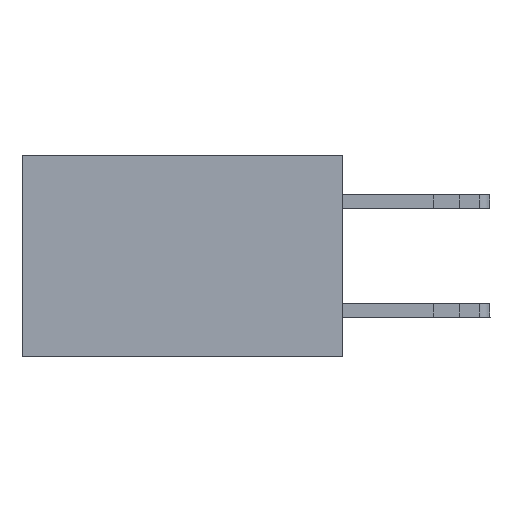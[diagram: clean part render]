
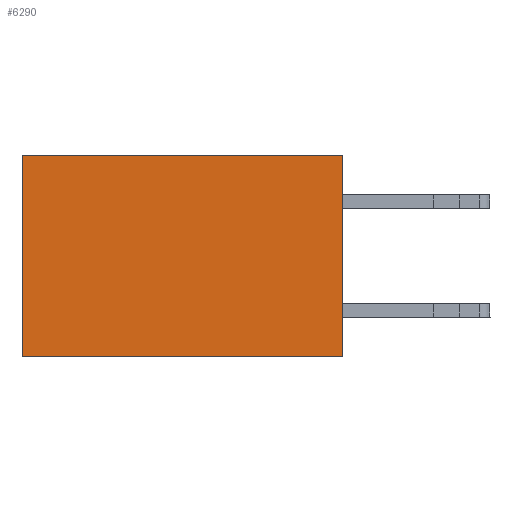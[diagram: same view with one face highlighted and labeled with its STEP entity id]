
A CAD part, left-side view. The second image highlights one B-rep face of the part: STEP entity #6290.
In plain terms, the highlighted planar face has unit normal (-1, 0, 0).
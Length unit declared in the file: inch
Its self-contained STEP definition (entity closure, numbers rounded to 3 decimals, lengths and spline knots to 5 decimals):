
#499 = DIRECTION ( 'NONE',  ( 0., 0., -1. ) ) ;
#519 = DIRECTION ( 'NONE',  ( 0., 0., -1. ) ) ;
#603 = DIRECTION ( 'NONE',  ( 1., 0., 0. ) ) ;
#666 = CARTESIAN_POINT ( 'NONE',  ( 0.277, 0., -0.37 ) ) ;
#763 = PLANE ( 'NONE',  #25191 ) ;
#1159 = VECTOR ( 'NONE', #11105, 39.37008 ) ;
#1438 = ORIENTED_EDGE ( 'NONE', *, *, #6607, .F. ) ;
#1777 = EDGE_CURVE ( 'NONE', #17716, #19414, #12972, .T. ) ;
#3686 = LINE ( 'NONE', #11729, #23177 ) ;
#4173 = ORIENTED_EDGE ( 'NONE', *, *, #1777, .F. ) ;
#4910 = FACE_OUTER_BOUND ( 'NONE', #6240, .T. ) ;
#5058 = VERTEX_POINT ( 'NONE', #5204 ) ;
#5204 = CARTESIAN_POINT ( 'NONE',  ( 0.277, 0.59, 0. ) ) ;
#5438 = CARTESIAN_POINT ( 'NONE',  ( 0.277, 0., 0. ) ) ;
#6240 = EDGE_LOOP ( 'NONE', ( #19880, #1438, #4173, #17797 ) ) ;
#6290 = ADVANCED_FACE ( 'NONE', ( #4910 ), #763, .F. ) ;
#6607 = EDGE_CURVE ( 'NONE', #19414, #14735, #19266, .T. ) ;
#6634 = LINE ( 'NONE', #21291, #23397 ) ;
#11105 = DIRECTION ( 'NONE',  ( 0., 1., 0. ) ) ;
#11729 = CARTESIAN_POINT ( 'NONE',  ( 0.277, 0., 0. ) ) ;
#12972 = LINE ( 'NONE', #25858, #23944 ) ;
#13496 = CARTESIAN_POINT ( 'NONE',  ( 0.277, 0., -0.37 ) ) ;
#13923 = DIRECTION ( 'NONE',  ( 0., 1., 0. ) ) ;
#14735 = VERTEX_POINT ( 'NONE', #27797 ) ;
#16822 = DIRECTION ( 'NONE',  ( 0., 0., -1. ) ) ;
#17716 = VERTEX_POINT ( 'NONE', #5438 ) ;
#17797 = ORIENTED_EDGE ( 'NONE', *, *, #21143, .T. ) ;
#19266 = LINE ( 'NONE', #13496, #1159 ) ;
#19414 = VERTEX_POINT ( 'NONE', #19454 ) ;
#19454 = CARTESIAN_POINT ( 'NONE',  ( 0.277, 0., -0.37 ) ) ;
#19880 = ORIENTED_EDGE ( 'NONE', *, *, #26617, .T. ) ;
#21143 = EDGE_CURVE ( 'NONE', #17716, #5058, #3686, .T. ) ;
#21291 = CARTESIAN_POINT ( 'NONE',  ( 0.277, 0.59, -0.37 ) ) ;
#23177 = VECTOR ( 'NONE', #13923, 39.37008 ) ;
#23397 = VECTOR ( 'NONE', #16822, 39.37008 ) ;
#23944 = VECTOR ( 'NONE', #499, 39.37008 ) ;
#25191 = AXIS2_PLACEMENT_3D ( 'NONE', #666, #603, #519 ) ;
#25858 = CARTESIAN_POINT ( 'NONE',  ( 0.277, 0., -0.37 ) ) ;
#26617 = EDGE_CURVE ( 'NONE', #5058, #14735, #6634, .T. ) ;
#27797 = CARTESIAN_POINT ( 'NONE',  ( 0.277, 0.59, -0.37 ) ) ;
